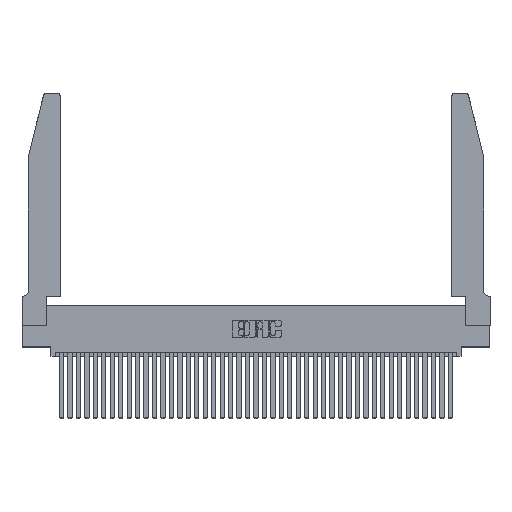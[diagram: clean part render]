
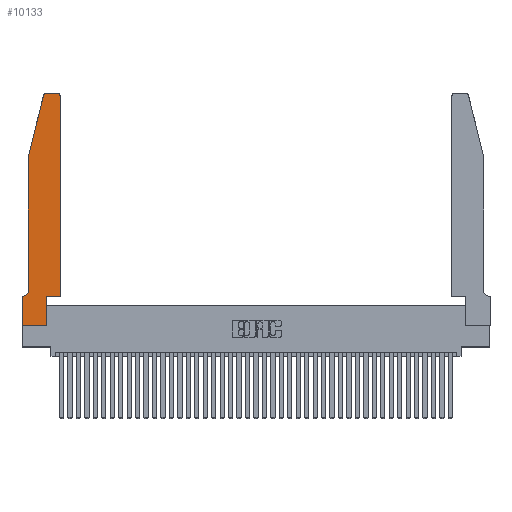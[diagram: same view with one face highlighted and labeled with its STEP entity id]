
A CAD part, top view. The second image highlights one B-rep face of the part: STEP entity #10133.
In plain terms, the highlighted planar face has unit normal (0, 0, 1).
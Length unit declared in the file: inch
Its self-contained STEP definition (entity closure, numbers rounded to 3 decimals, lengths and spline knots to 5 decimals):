
#557 = EDGE_CURVE ( 'NONE', #38281, #3706, #13715, .T. ) ;
#869 = LINE ( 'NONE', #23343, #16240 ) ;
#1062 = ORIENTED_EDGE ( 'NONE', *, *, #30640, .T. ) ;
#2380 = CARTESIAN_POINT ( 'NONE',  ( 0.0055, 0.35, 0.37 ) ) ;
#2412 = LINE ( 'NONE', #40645, #21694 ) ;
#3706 = VERTEX_POINT ( 'NONE', #29956 ) ;
#4878 = DIRECTION ( 'NONE',  ( -0.239, -0.971, 0. ) ) ;
#5216 = CARTESIAN_POINT ( 'NONE',  ( 0., 0.35, 0.37 ) ) ;
#5323 = EDGE_CURVE ( 'NONE', #27026, #38281, #869, .T. ) ;
#5455 = DIRECTION ( 'NONE',  ( 0., 0., 1. ) ) ;
#5499 = VECTOR ( 'NONE', #10384, 39.37008 ) ;
#5559 = CARTESIAN_POINT ( 'NONE',  ( 0.0755, 0.42, 0.37 ) ) ;
#5734 = ORIENTED_EDGE ( 'NONE', *, *, #10649, .T. ) ;
#5803 = DIRECTION ( 'NONE',  ( -1., 0., 0. ) ) ;
#6127 = CIRCLE ( 'NONE', #25613, 0.03 ) ;
#7770 = CARTESIAN_POINT ( 'NONE',  ( 0.2605, 2.75, 0.37 ) ) ;
#7990 = EDGE_CURVE ( 'NONE', #38492, #32127, #6127, .T. ) ;
#8078 = EDGE_CURVE ( 'NONE', #40004, #25694, #16975, .T. ) ;
#8467 = ORIENTED_EDGE ( 'NONE', *, *, #5323, .T. ) ;
#8590 = CARTESIAN_POINT ( 'NONE',  ( 0.2865, 0., 0.37 ) ) ;
#8612 = DIRECTION ( 'NONE',  ( 1., 0., 0. ) ) ;
#10133 = ADVANCED_FACE ( 'NONE', ( #33035 ), #26910, .T. ) ;
#10384 = DIRECTION ( 'NONE',  ( -1., 0., 0. ) ) ;
#10649 = EDGE_CURVE ( 'NONE', #22388, #29218, #37010, .T. ) ;
#10940 = CARTESIAN_POINT ( 'NONE',  ( 0.2865, 0.35, 0.37 ) ) ;
#11339 = ORIENTED_EDGE ( 'NONE', *, *, #7990, .T. ) ;
#11625 = CARTESIAN_POINT ( 'NONE',  ( 0.0755, 2., 0.37 ) ) ;
#12116 = CARTESIAN_POINT ( 'NONE',  ( 0.284, 2.75, 0.37 ) ) ;
#12442 = CARTESIAN_POINT ( 'NONE',  ( 0.4505, 0.35, 0.37 ) ) ;
#12834 = DIRECTION ( 'NONE',  ( 0., 0., 1. ) ) ;
#13057 = VECTOR ( 'NONE', #15658, 39.37008 ) ;
#13435 = DIRECTION ( 'NONE',  ( 0., -1., 0. ) ) ;
#13715 = LINE ( 'NONE', #10940, #31156 ) ;
#13821 = ORIENTED_EDGE ( 'NONE', *, *, #557, .T. ) ;
#13856 = CARTESIAN_POINT ( 'NONE',  ( 0., 0.35, 0.37 ) ) ;
#14642 = CARTESIAN_POINT ( 'NONE',  ( 0.4505, 0.35, 0.37 ) ) ;
#15658 = DIRECTION ( 'NONE',  ( 1., 0., 0. ) ) ;
#15907 = VERTEX_POINT ( 'NONE', #2380 ) ;
#15921 = CARTESIAN_POINT ( 'NONE',  ( 0.4505, 2.72, 0.37 ) ) ;
#16240 = VECTOR ( 'NONE', #19683, 39.37008 ) ;
#16437 = EDGE_CURVE ( 'NONE', #39133, #38492, #18789, .T. ) ;
#16797 = VECTOR ( 'NONE', #34364, 39.37008 ) ;
#16975 = CIRCLE ( 'NONE', #23242, 0.03 ) ;
#18470 = CARTESIAN_POINT ( 'NONE',  ( 0.0055, 0.42, 0.37 ) ) ;
#18685 = CARTESIAN_POINT ( 'NONE',  ( 0.284, 2.72, 0.37 ) ) ;
#18789 = LINE ( 'NONE', #28031, #16797 ) ;
#19487 = LINE ( 'NONE', #12442, #13057 ) ;
#19600 = ORIENTED_EDGE ( 'NONE', *, *, #25881, .T. ) ;
#19683 = DIRECTION ( 'NONE',  ( 1., 0., 0. ) ) ;
#19929 = AXIS2_PLACEMENT_3D ( 'NONE', #18470, #31252, #5803 ) ;
#20698 = DIRECTION ( 'NONE',  ( 0., 1., 0. ) ) ;
#20930 = CARTESIAN_POINT ( 'NONE',  ( 0.4205, 2.75, 0.37 ) ) ;
#21689 = DIRECTION ( 'NONE',  ( -1., 0., 0. ) ) ;
#21694 = VECTOR ( 'NONE', #21689, 39.37008 ) ;
#22363 = ORIENTED_EDGE ( 'NONE', *, *, #8078, .T. ) ;
#22388 = VERTEX_POINT ( 'NONE', #11625 ) ;
#23112 = VECTOR ( 'NONE', #29630, 39.37008 ) ;
#23242 = AXIS2_PLACEMENT_3D ( 'NONE', #18685, #27591, #8612 ) ;
#23343 = CARTESIAN_POINT ( 'NONE',  ( 0., 0., 0.37 ) ) ;
#23985 = CARTESIAN_POINT ( 'NONE',  ( 0.0755, 2., 0.37 ) ) ;
#25079 = DIRECTION ( 'NONE',  ( 1., 0., 0. ) ) ;
#25281 = CARTESIAN_POINT ( 'NONE',  ( 0.25487, 2.72718, 0.37 ) ) ;
#25589 = VERTEX_POINT ( 'NONE', #5216 ) ;
#25613 = AXIS2_PLACEMENT_3D ( 'NONE', #31066, #5455, #31335 ) ;
#25694 = VERTEX_POINT ( 'NONE', #25281 ) ;
#25756 = CARTESIAN_POINT ( 'NONE',  ( 0.0755, 2., 0.37 ) ) ;
#25881 = EDGE_CURVE ( 'NONE', #25694, #22388, #26061, .T. ) ;
#26061 = LINE ( 'NONE', #23985, #38480 ) ;
#26155 = CARTESIAN_POINT ( 'NONE',  ( 0., 0., 0.37 ) ) ;
#26193 = CARTESIAN_POINT ( 'NONE',  ( 0., 0., 0.37 ) ) ;
#26479 = EDGE_CURVE ( 'NONE', #25589, #27026, #26516, .T. ) ;
#26516 = LINE ( 'NONE', #26193, #34505 ) ;
#26910 = PLANE ( 'NONE',  #32826 ) ;
#27026 = VERTEX_POINT ( 'NONE', #26155 ) ;
#27071 = CIRCLE ( 'NONE', #19929, 0.07 ) ;
#27591 = DIRECTION ( 'NONE',  ( 0., 0., 1. ) ) ;
#28031 = CARTESIAN_POINT ( 'NONE',  ( 0.4505, 0.35, 0.37 ) ) ;
#28042 = ORIENTED_EDGE ( 'NONE', *, *, #32798, .T. ) ;
#29218 = VERTEX_POINT ( 'NONE', #5559 ) ;
#29630 = DIRECTION ( 'NONE',  ( 0., -1., 0. ) ) ;
#29956 = CARTESIAN_POINT ( 'NONE',  ( 0.2865, 0.35, 0.37 ) ) ;
#30640 = EDGE_CURVE ( 'NONE', #32127, #40004, #36696, .T. ) ;
#31066 = CARTESIAN_POINT ( 'NONE',  ( 0.4205, 2.72, 0.37 ) ) ;
#31156 = VECTOR ( 'NONE', #20698, 39.37008 ) ;
#31252 = DIRECTION ( 'NONE',  ( 0., 0., -1. ) ) ;
#31335 = DIRECTION ( 'NONE',  ( 1., 0., 0. ) ) ;
#31405 = ORIENTED_EDGE ( 'NONE', *, *, #26479, .T. ) ;
#32127 = VERTEX_POINT ( 'NONE', #20930 ) ;
#32650 = ORIENTED_EDGE ( 'NONE', *, *, #16437, .T. ) ;
#32798 = EDGE_CURVE ( 'NONE', #29218, #15907, #27071, .T. ) ;
#32826 = AXIS2_PLACEMENT_3D ( 'NONE', #13856, #12834, #25079 ) ;
#33035 = FACE_OUTER_BOUND ( 'NONE', #34446, .T. ) ;
#33802 = ORIENTED_EDGE ( 'NONE', *, *, #40012, .T. ) ;
#34120 = EDGE_CURVE ( 'NONE', #3706, #39133, #19487, .T. ) ;
#34364 = DIRECTION ( 'NONE',  ( 0., 1., 0. ) ) ;
#34446 = EDGE_LOOP ( 'NONE', ( #1062, #22363, #19600, #5734, #28042, #33802, #31405, #8467, #13821, #40653, #32650, #11339 ) ) ;
#34505 = VECTOR ( 'NONE', #13435, 39.37008 ) ;
#36696 = LINE ( 'NONE', #7770, #5499 ) ;
#37010 = LINE ( 'NONE', #25756, #23112 ) ;
#38281 = VERTEX_POINT ( 'NONE', #8590 ) ;
#38480 = VECTOR ( 'NONE', #4878, 39.37008 ) ;
#38492 = VERTEX_POINT ( 'NONE', #15921 ) ;
#39133 = VERTEX_POINT ( 'NONE', #14642 ) ;
#40004 = VERTEX_POINT ( 'NONE', #12116 ) ;
#40012 = EDGE_CURVE ( 'NONE', #15907, #25589, #2412, .T. ) ;
#40645 = CARTESIAN_POINT ( 'NONE',  ( 0.0755, 0.35, 0.37 ) ) ;
#40653 = ORIENTED_EDGE ( 'NONE', *, *, #34120, .T. ) ;
